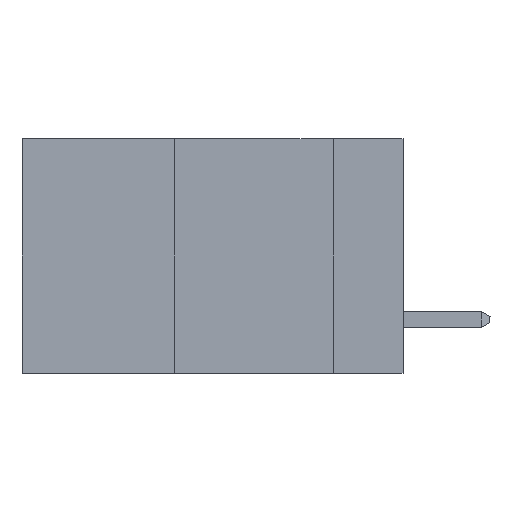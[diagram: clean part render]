
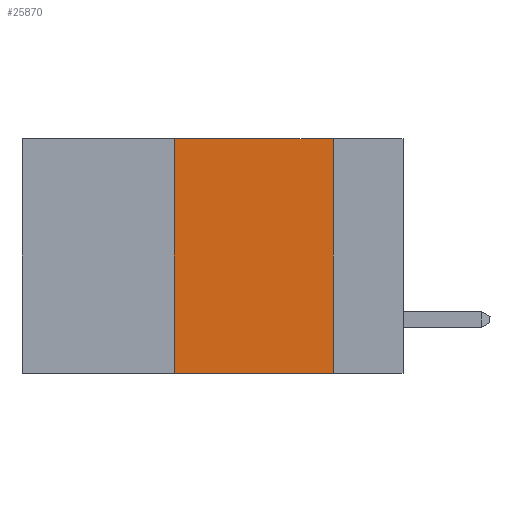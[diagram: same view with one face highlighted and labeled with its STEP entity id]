
A CAD part, left-side view. The second image highlights one B-rep face of the part: STEP entity #25870.
In plain terms, the highlighted planar face has unit normal (-1, 0, 0).
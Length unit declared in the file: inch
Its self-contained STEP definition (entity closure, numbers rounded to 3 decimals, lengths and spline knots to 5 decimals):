
#530 = CARTESIAN_POINT ( 'NONE',  ( 0., 0.6, 0. ) ) ;
#2425 = VECTOR ( 'NONE', #15996, 39.37008 ) ;
#2809 = LINE ( 'NONE', #11324, #2425 ) ;
#4272 = CARTESIAN_POINT ( 'NONE',  ( 0., 0.36, -0.37 ) ) ;
#4488 = ORIENTED_EDGE ( 'NONE', *, *, #9136, .F. ) ;
#9136 = EDGE_CURVE ( 'NONE', #37178, #30363, #40252, .T. ) ;
#9159 = LINE ( 'NONE', #12215, #18686 ) ;
#9295 = EDGE_CURVE ( 'NONE', #30363, #15105, #2809, .T. ) ;
#11324 = CARTESIAN_POINT ( 'NONE',  ( 0., 0.11, 0. ) ) ;
#11709 = CARTESIAN_POINT ( 'NONE',  ( 0., 0.11, -0.37 ) ) ;
#12215 = CARTESIAN_POINT ( 'NONE',  ( 0., 0.36, 0. ) ) ;
#14340 = CARTESIAN_POINT ( 'NONE',  ( 0., 0.11, 0. ) ) ;
#15105 = VERTEX_POINT ( 'NONE', #11709 ) ;
#15996 = DIRECTION ( 'NONE',  ( 0., 0., -1. ) ) ;
#16515 = PLANE ( 'NONE',  #28990 ) ;
#18686 = VECTOR ( 'NONE', #29043, 39.37008 ) ;
#19144 = DIRECTION ( 'NONE',  ( 0., 0., -1. ) ) ;
#20448 = LINE ( 'NONE', #29945, #32448 ) ;
#21063 = VECTOR ( 'NONE', #29917, 39.37008 ) ;
#25812 = CARTESIAN_POINT ( 'NONE',  ( 0., 0.6, 0. ) ) ;
#25870 = ADVANCED_FACE ( 'NONE', ( #37911 ), #16515, .F. ) ;
#28990 = AXIS2_PLACEMENT_3D ( 'NONE', #25812, #29046, #19144 ) ;
#29043 = DIRECTION ( 'NONE',  ( 0., 0., 1. ) ) ;
#29046 = DIRECTION ( 'NONE',  ( 1., 0., 0. ) ) ;
#29917 = DIRECTION ( 'NONE',  ( 0., -1., 0. ) ) ;
#29945 = CARTESIAN_POINT ( 'NONE',  ( 0., 0.6, -0.37 ) ) ;
#30363 = VERTEX_POINT ( 'NONE', #14340 ) ;
#30662 = ORIENTED_EDGE ( 'NONE', *, *, #39816, .F. ) ;
#31223 = VERTEX_POINT ( 'NONE', #4272 ) ;
#31869 = ORIENTED_EDGE ( 'NONE', *, *, #9295, .F. ) ;
#32448 = VECTOR ( 'NONE', #37077, 39.37008 ) ;
#34279 = ORIENTED_EDGE ( 'NONE', *, *, #39496, .T. ) ;
#34535 = EDGE_LOOP ( 'NONE', ( #31869, #4488, #30662, #34279 ) ) ;
#37077 = DIRECTION ( 'NONE',  ( 0., -1., 0. ) ) ;
#37178 = VERTEX_POINT ( 'NONE', #40907 ) ;
#37911 = FACE_OUTER_BOUND ( 'NONE', #34535, .T. ) ;
#39496 = EDGE_CURVE ( 'NONE', #31223, #15105, #20448, .T. ) ;
#39816 = EDGE_CURVE ( 'NONE', #31223, #37178, #9159, .T. ) ;
#40252 = LINE ( 'NONE', #530, #21063 ) ;
#40907 = CARTESIAN_POINT ( 'NONE',  ( 0., 0.36, 0. ) ) ;
